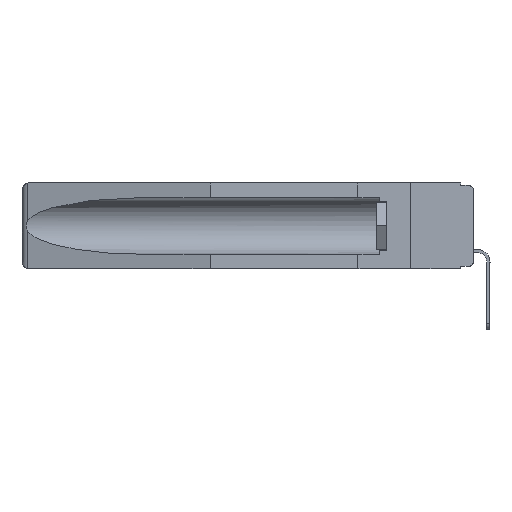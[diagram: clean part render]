
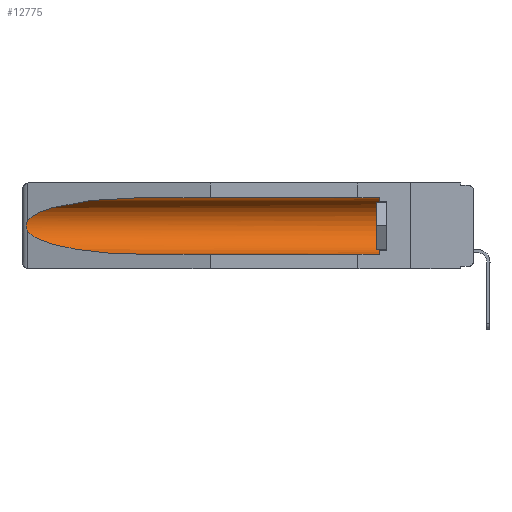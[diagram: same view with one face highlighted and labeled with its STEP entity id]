
A CAD part, left-side view. The second image highlights one B-rep face of the part: STEP entity #12775.
In plain terms, the highlighted cylindrical face has radius 2.857 mm (diameter 5.715 mm), a partial arc.
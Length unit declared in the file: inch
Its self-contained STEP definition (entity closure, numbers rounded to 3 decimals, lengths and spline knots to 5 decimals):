
#617 = CARTESIAN_POINT ( 'NONE',  ( 0.26537, 1.52718, -0.19328 ) ) ;
#703 = ORIENTED_EDGE ( 'NONE', *, *, #14904, .T. ) ;
#1003 = ORIENTED_EDGE ( 'NONE', *, *, #4460, .T. ) ;
#1233 = EDGE_LOOP ( 'NONE', ( #1003, #4007, #20580, #4638, #703, #17513 ) ) ;
#1566 = CARTESIAN_POINT ( 'NONE',  ( 0.155, 1.07973, -0.284 ) ) ;
#1651 =( BOUNDED_CURVE ( )  B_SPLINE_CURVE ( 3, ( #18646, #20354, #11320, #1566 ),
 .UNSPECIFIED., .F., .T. ) 
 B_SPLINE_CURVE_WITH_KNOTS ( ( 4, 4 ),
 ( 0.1948, 1.5708 ),
 .UNSPECIFIED. ) 
 CURVE ( )  GEOMETRIC_REPRESENTATION_ITEM ( )  RATIONAL_B_SPLINE_CURVE ( ( 1., 0.848, 0.848, 1. ) ) 
 REPRESENTATION_ITEM ( '' )  );
#2307 = VERTEX_POINT ( 'NONE', #14484 ) ;
#2393 = CARTESIAN_POINT ( 'NONE',  ( 0.155, -0.30754, -0.1715 ) ) ;
#2452 = CARTESIAN_POINT ( 'NONE',  ( 0.26597, 1.5296, -0.19026 ) ) ;
#2821 = CARTESIAN_POINT ( 'NONE',  ( 0.26537, 1.52718, -0.14972 ) ) ;
#3543 = B_SPLINE_CURVE_WITH_KNOTS ( 'NONE', 3,
 ( #17779, #16174, #11952, #13708, #4213, #19505, #23501, #23389, #2452, #15925 ),
 .UNSPECIFIED., .F., .F.,
 ( 4, 2, 2, 2, 4 ),
 ( 0., 0.00029, 0.00058, 0.00087, 0.00117 ),
 .UNSPECIFIED. ) ;
#4007 = ORIENTED_EDGE ( 'NONE', *, *, #7220, .T. ) ;
#4213 = CARTESIAN_POINT ( 'NONE',  ( 0.2675, 1.53308, -0.16763 ) ) ;
#4222 = CIRCLE ( 'NONE', #5808, 0.1125 ) ;
#4460 = EDGE_CURVE ( 'NONE', #13654, #22744, #7352, .T. ) ;
#4555 = CARTESIAN_POINT ( 'NONE',  ( 0.155, 0.126, -0.1715 ) ) ;
#4638 = ORIENTED_EDGE ( 'NONE', *, *, #7385, .F. ) ;
#5808 = AXIS2_PLACEMENT_3D ( 'NONE', #4555, #21348, #10179 ) ;
#6785 = VERTEX_POINT ( 'NONE', #617 ) ;
#7220 = EDGE_CURVE ( 'NONE', #22744, #6785, #3543, .T. ) ;
#7352 =( BOUNDED_CURVE ( )  B_SPLINE_CURVE ( 3, ( #15573, #19654, #23153, #13732 ),
 .UNSPECIFIED., .F., .T. ) 
 B_SPLINE_CURVE_WITH_KNOTS ( ( 4, 4 ),
 ( 4.71239, 6.08839 ),
 .UNSPECIFIED. ) 
 CURVE ( )  GEOMETRIC_REPRESENTATION_ITEM ( )  RATIONAL_B_SPLINE_CURVE ( ( 1., 0.848, 0.848, 1. ) ) 
 REPRESENTATION_ITEM ( '' )  );
#7385 = EDGE_CURVE ( 'NONE', #2307, #10496, #20363, .T. ) ;
#9770 = DIRECTION ( 'NONE',  ( 0., 1., 0. ) ) ;
#10179 = DIRECTION ( 'NONE',  ( 0., 0., 1. ) ) ;
#10496 = VERTEX_POINT ( 'NONE', #11719 ) ;
#11320 = CARTESIAN_POINT ( 'NONE',  ( 0.21114, 1.30732, -0.284 ) ) ;
#11380 = AXIS2_PLACEMENT_3D ( 'NONE', #2393, #9770, #19692 ) ;
#11719 = CARTESIAN_POINT ( 'NONE',  ( 0.155, 1.07973, -0.284 ) ) ;
#11952 = CARTESIAN_POINT ( 'NONE',  ( 0.26654, 1.53092, -0.15636 ) ) ;
#12170 = CARTESIAN_POINT ( 'NONE',  ( 0.155, 1.07973, -0.059 ) ) ;
#12775 = ADVANCED_FACE ( 'NONE', ( #19205 ), #17469, .F. ) ;
#13120 = CARTESIAN_POINT ( 'NONE',  ( 0.155, -0.30754, -0.059 ) ) ;
#13654 = VERTEX_POINT ( 'NONE', #12170 ) ;
#13708 = CARTESIAN_POINT ( 'NONE',  ( 0.2673, 1.5327, -0.16383 ) ) ;
#13732 = CARTESIAN_POINT ( 'NONE',  ( 0.26537, 1.52718, -0.14972 ) ) ;
#14484 = CARTESIAN_POINT ( 'NONE',  ( 0.155, 0.126, -0.284 ) ) ;
#14708 = EDGE_CURVE ( 'NONE', #15748, #13654, #24152, .T. ) ;
#14904 = EDGE_CURVE ( 'NONE', #2307, #15748, #4222, .T. ) ;
#15573 = CARTESIAN_POINT ( 'NONE',  ( 0.155, 1.07973, -0.059 ) ) ;
#15748 = VERTEX_POINT ( 'NONE', #17555 ) ;
#15925 = CARTESIAN_POINT ( 'NONE',  ( 0.26537, 1.52718, -0.19328 ) ) ;
#16174 = CARTESIAN_POINT ( 'NONE',  ( 0.26597, 1.52961, -0.15275 ) ) ;
#16660 = CARTESIAN_POINT ( 'NONE',  ( 0.155, -0.30754, -0.284 ) ) ;
#16996 = VECTOR ( 'NONE', #18526, 39.37008 ) ;
#17469 = CYLINDRICAL_SURFACE ( 'NONE', #11380, 0.1125 ) ;
#17513 = ORIENTED_EDGE ( 'NONE', *, *, #14708, .T. ) ;
#17555 = CARTESIAN_POINT ( 'NONE',  ( 0.155, 0.126, -0.059 ) ) ;
#17779 = CARTESIAN_POINT ( 'NONE',  ( 0.26537, 1.52718, -0.14972 ) ) ;
#18448 = EDGE_CURVE ( 'NONE', #6785, #10496, #1651, .T. ) ;
#18526 = DIRECTION ( 'NONE',  ( 0., 1., 0. ) ) ;
#18646 = CARTESIAN_POINT ( 'NONE',  ( 0.26537, 1.52718, -0.19328 ) ) ;
#18794 = DIRECTION ( 'NONE',  ( 0., 1., 0. ) ) ;
#19205 = FACE_OUTER_BOUND ( 'NONE', #1233, .T. ) ;
#19328 = VECTOR ( 'NONE', #18794, 39.37008 ) ;
#19505 = CARTESIAN_POINT ( 'NONE',  ( 0.2675, 1.53308, -0.17534 ) ) ;
#19654 = CARTESIAN_POINT ( 'NONE',  ( 0.21114, 1.30732, -0.059 ) ) ;
#19692 = DIRECTION ( 'NONE',  ( 0., 0., 1. ) ) ;
#20354 = CARTESIAN_POINT ( 'NONE',  ( 0.25451, 1.48313, -0.24835 ) ) ;
#20363 = LINE ( 'NONE', #16660, #16996 ) ;
#20580 = ORIENTED_EDGE ( 'NONE', *, *, #18448, .T. ) ;
#21348 = DIRECTION ( 'NONE',  ( 0., -1., 0. ) ) ;
#22744 = VERTEX_POINT ( 'NONE', #2821 ) ;
#23153 = CARTESIAN_POINT ( 'NONE',  ( 0.25451, 1.48313, -0.09465 ) ) ;
#23389 = CARTESIAN_POINT ( 'NONE',  ( 0.26655, 1.53094, -0.18657 ) ) ;
#23501 = CARTESIAN_POINT ( 'NONE',  ( 0.2673, 1.53269, -0.17917 ) ) ;
#24152 = LINE ( 'NONE', #13120, #19328 ) ;
